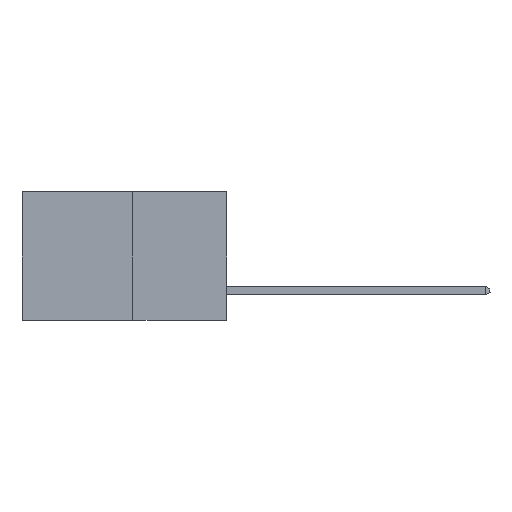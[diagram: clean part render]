
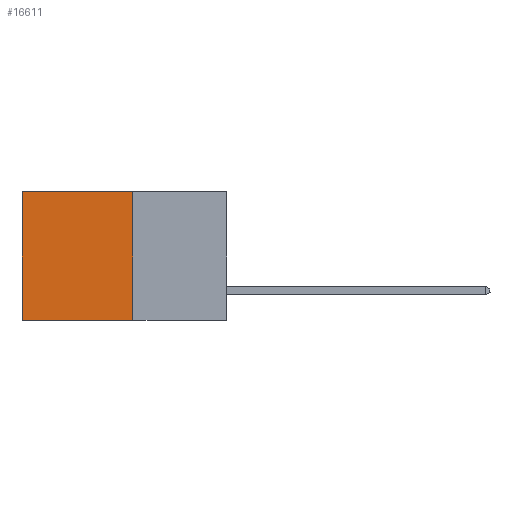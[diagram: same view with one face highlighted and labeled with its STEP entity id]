
A CAD part, left-side view. The second image highlights one B-rep face of the part: STEP entity #16611.
In plain terms, the highlighted planar face has unit normal (-1, 0, 0).
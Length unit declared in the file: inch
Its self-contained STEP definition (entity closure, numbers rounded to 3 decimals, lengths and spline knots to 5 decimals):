
#367 = ORIENTED_EDGE ( 'NONE', *, *, #13094, .T. ) ;
#4622 = CARTESIAN_POINT ( 'NONE',  ( 0.277, 0.27, -0.37 ) ) ;
#6029 = FACE_OUTER_BOUND ( 'NONE', #21514, .T. ) ;
#6531 = VERTEX_POINT ( 'NONE', #15146 ) ;
#6584 = VECTOR ( 'NONE', #15180, 39.37008 ) ;
#6659 = CARTESIAN_POINT ( 'NONE',  ( 0.277, 0.27, -0.37 ) ) ;
#7130 = AXIS2_PLACEMENT_3D ( 'NONE', #6659, #23625, #9051 ) ;
#7230 = DIRECTION ( 'NONE',  ( 0., 1., 0. ) ) ;
#7772 = VECTOR ( 'NONE', #9165, 39.37008 ) ;
#9051 = DIRECTION ( 'NONE',  ( 0., 0., -1. ) ) ;
#9165 = DIRECTION ( 'NONE',  ( 0., 0., -1. ) ) ;
#9537 = CARTESIAN_POINT ( 'NONE',  ( 0.277, 0.27, 0. ) ) ;
#10591 = VERTEX_POINT ( 'NONE', #23965 ) ;
#10956 = LINE ( 'NONE', #4622, #18234 ) ;
#11203 = VERTEX_POINT ( 'NONE', #19400 ) ;
#11287 = LINE ( 'NONE', #9537, #22755 ) ;
#12725 = CARTESIAN_POINT ( 'NONE',  ( 0.277, 0.27, -0.37 ) ) ;
#12958 = LINE ( 'NONE', #12725, #6584 ) ;
#13094 = EDGE_CURVE ( 'NONE', #17296, #10591, #20726, .T. ) ;
#15146 = CARTESIAN_POINT ( 'NONE',  ( 0.277, 0.27, 0. ) ) ;
#15180 = DIRECTION ( 'NONE',  ( 0., 0., -1. ) ) ;
#15790 = EDGE_CURVE ( 'NONE', #11203, #10591, #10956, .T. ) ;
#16611 = ADVANCED_FACE ( 'NONE', ( #6029 ), #18763, .F. ) ;
#16737 = ORIENTED_EDGE ( 'NONE', *, *, #20004, .F. ) ;
#17296 = VERTEX_POINT ( 'NONE', #30927 ) ;
#18234 = VECTOR ( 'NONE', #19149, 39.37008 ) ;
#18763 = PLANE ( 'NONE',  #7130 ) ;
#19149 = DIRECTION ( 'NONE',  ( 0., 1., 0. ) ) ;
#19400 = CARTESIAN_POINT ( 'NONE',  ( 0.277, 0.27, -0.37 ) ) ;
#20004 = EDGE_CURVE ( 'NONE', #6531, #11203, #12958, .T. ) ;
#20726 = LINE ( 'NONE', #23741, #7772 ) ;
#21069 = ORIENTED_EDGE ( 'NONE', *, *, #27391, .T. ) ;
#21514 = EDGE_LOOP ( 'NONE', ( #367, #27180, #16737, #21069 ) ) ;
#22755 = VECTOR ( 'NONE', #7230, 39.37008 ) ;
#23625 = DIRECTION ( 'NONE',  ( 1., 0., 0. ) ) ;
#23741 = CARTESIAN_POINT ( 'NONE',  ( 0.277, 0.59, -0.37 ) ) ;
#23965 = CARTESIAN_POINT ( 'NONE',  ( 0.277, 0.59, -0.37 ) ) ;
#27180 = ORIENTED_EDGE ( 'NONE', *, *, #15790, .F. ) ;
#27391 = EDGE_CURVE ( 'NONE', #6531, #17296, #11287, .T. ) ;
#30927 = CARTESIAN_POINT ( 'NONE',  ( 0.277, 0.59, 0. ) ) ;
